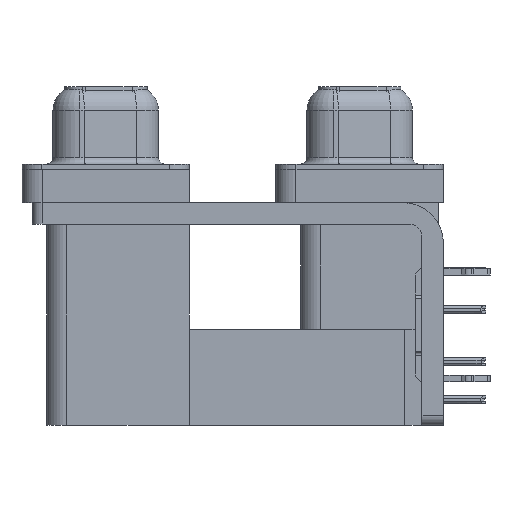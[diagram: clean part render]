
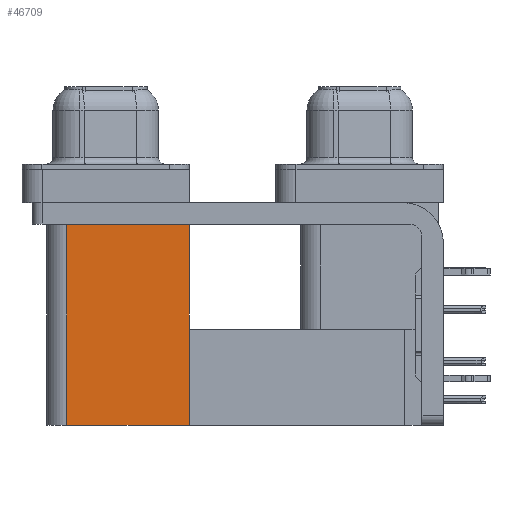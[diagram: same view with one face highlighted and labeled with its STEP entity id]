
A CAD part, left-side view. The second image highlights one B-rep face of the part: STEP entity #46709.
In plain terms, the highlighted planar face has unit normal (-1, 0, 0).
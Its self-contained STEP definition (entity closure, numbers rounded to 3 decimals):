
#1185 = EDGE_LOOP ( 'NONE', ( #19982, #45857, #11480, #22792 ) ) ;
#4417 = DIRECTION ( 'NONE',  ( 1., 0., 0. ) ) ;
#5118 = CARTESIAN_POINT ( 'NONE',  ( 3.765, 21.975, -2.5 ) ) ;
#7590 = DIRECTION ( 'NONE',  ( 0., 1., 0. ) ) ;
#7909 = PLANE ( 'NONE',  #29426 ) ;
#8745 = CARTESIAN_POINT ( 'NONE',  ( 3.765, 21.975, -19.2 ) ) ;
#9071 = DIRECTION ( 'NONE',  ( 0., 1., 0. ) ) ;
#11480 = ORIENTED_EDGE ( 'NONE', *, *, #25087, .F. ) ;
#14275 = VERTEX_POINT ( 'NONE', #5118 ) ;
#16428 = CARTESIAN_POINT ( 'NONE',  ( 3.765, 12.775, -19.2 ) ) ;
#18679 = CARTESIAN_POINT ( 'NONE',  ( 3.765, 12.775, -19.2 ) ) ;
#19269 = LINE ( 'NONE', #41543, #40629 ) ;
#19488 = VERTEX_POINT ( 'NONE', #22197 ) ;
#19982 = ORIENTED_EDGE ( 'NONE', *, *, #33309, .T. ) ;
#20088 = VERTEX_POINT ( 'NONE', #16428 ) ;
#20189 = DIRECTION ( 'NONE',  ( 0., 0., 1. ) ) ;
#21188 = VERTEX_POINT ( 'NONE', #32855 ) ;
#22197 = CARTESIAN_POINT ( 'NONE',  ( 3.765, 12.775, -2.5 ) ) ;
#22792 = ORIENTED_EDGE ( 'NONE', *, *, #42177, .T. ) ;
#23522 = CARTESIAN_POINT ( 'NONE',  ( 3.765, 12.775, -19.2 ) ) ;
#25087 = EDGE_CURVE ( 'NONE', #20088, #21188, #19269, .T. ) ;
#26640 = EDGE_CURVE ( 'NONE', #21188, #14275, #39475, .T. ) ;
#26840 = LINE ( 'NONE', #18679, #45143 ) ;
#29426 = AXIS2_PLACEMENT_3D ( 'NONE', #23522, #4417, #38628 ) ;
#32855 = CARTESIAN_POINT ( 'NONE',  ( 3.765, 21.975, -19.2 ) ) ;
#33309 = EDGE_CURVE ( 'NONE', #19488, #14275, #44016, .T. ) ;
#38234 = DIRECTION ( 'NONE',  ( 0., 0., 1. ) ) ;
#38391 = FACE_OUTER_BOUND ( 'NONE', #1185, .T. ) ;
#38628 = DIRECTION ( 'NONE',  ( 0., 0., -1. ) ) ;
#38927 = VECTOR ( 'NONE', #20189, 1000. ) ;
#39475 = LINE ( 'NONE', #8745, #38927 ) ;
#39995 = VECTOR ( 'NONE', #9071, 1000. ) ;
#40629 = VECTOR ( 'NONE', #7590, 1000. ) ;
#41543 = CARTESIAN_POINT ( 'NONE',  ( 3.765, 12.775, -19.2 ) ) ;
#42177 = EDGE_CURVE ( 'NONE', #20088, #19488, #26840, .T. ) ;
#44016 = LINE ( 'NONE', #47996, #39995 ) ;
#45143 = VECTOR ( 'NONE', #38234, 1000. ) ;
#45857 = ORIENTED_EDGE ( 'NONE', *, *, #26640, .F. ) ;
#46709 = ADVANCED_FACE ( 'NONE', ( #38391 ), #7909, .F. ) ;
#47996 = CARTESIAN_POINT ( 'NONE',  ( 3.765, 12.775, -2.5 ) ) ;
